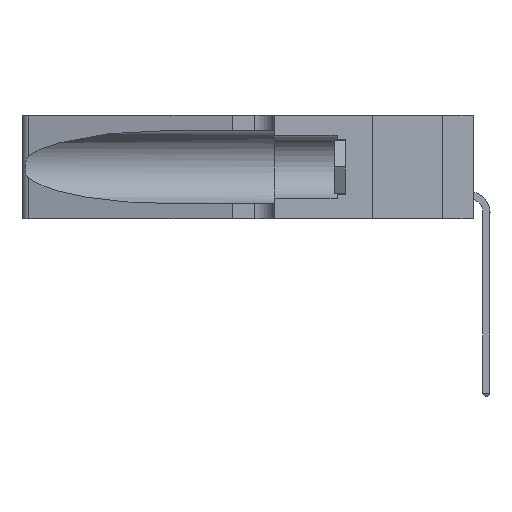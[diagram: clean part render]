
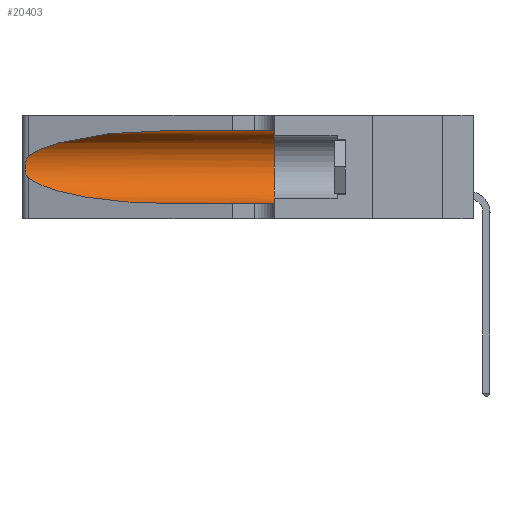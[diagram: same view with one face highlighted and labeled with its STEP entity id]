
A CAD part, left-side view. The second image highlights one B-rep face of the part: STEP entity #20403.
In plain terms, the highlighted cylindrical face has radius 3.308 mm (diameter 6.617 mm), a partial arc.
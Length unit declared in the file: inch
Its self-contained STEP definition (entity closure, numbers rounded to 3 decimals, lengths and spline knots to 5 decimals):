
#1357 = CARTESIAN_POINT ( 'NONE',  ( 0.1305, 1.61858, 0.31525 ) ) ;
#1443 =( BOUNDED_CURVE ( )  B_SPLINE_CURVE ( 3, ( #39841, #32537, #13638, #20014 ),
 .UNSPECIFIED., .F., .F. ) 
 B_SPLINE_CURVE_WITH_KNOTS ( ( 4, 4 ),
 ( 3.44316, 4.71239 ),
 .UNSPECIFIED. ) 
 CURVE ( )  GEOMETRIC_REPRESENTATION_ITEM ( )  RATIONAL_B_SPLINE_CURVE ( ( 1., 0.87, 0.87, 1. ) ) 
 REPRESENTATION_ITEM ( '' )  );
#2177 = DIRECTION ( 'NONE',  ( 0., -1., 0. ) ) ;
#2722 = CARTESIAN_POINT ( 'NONE',  ( 0.2373, 1.15595, 0.28018 ) ) ;
#2721 = CARTESIAN_POINT ( 'NONE',  ( 0.1305, 1.61858, 0.05475 ) ) ;
#4107 = EDGE_CURVE ( 'NONE', #25754, #6653, #5802, .T. ) ;
#4932 = VECTOR ( 'NONE', #26625, 39.37008 ) ;
#5802 =( BOUNDED_CURVE ( )  B_SPLINE_CURVE ( 3, ( #9171, #18716, #2722, #34427 ),
 .UNSPECIFIED., .F., .T. ) 
 B_SPLINE_CURVE_WITH_KNOTS ( ( 4, 4 ),
 ( 1.5708, 2.84003 ),
 .UNSPECIFIED. ) 
 CURVE ( )  GEOMETRIC_REPRESENTATION_ITEM ( )  RATIONAL_B_SPLINE_CURVE ( ( 1., 0.87, 0.87, 1. ) ) 
 REPRESENTATION_ITEM ( '' )  );
#6556 = CARTESIAN_POINT ( 'NONE',  ( 0.25639, 1.23186, 0.15144 ) ) ;
#6653 = VERTEX_POINT ( 'NONE', #25644 ) ;
#8670 = CARTESIAN_POINT ( 'NONE',  ( 0.26018, 1.23835, 0.19895 ) ) ;
#8811 = CARTESIAN_POINT ( 'NONE',  ( 0.26075, 1.23896, 0.178 ) ) ;
#8967 = AXIS2_PLACEMENT_3D ( 'NONE', #35806, #18061, #27048 ) ;
#9171 = CARTESIAN_POINT ( 'NONE',  ( 0.1305, 0.72297, 0.31525 ) ) ;
#10238 = CARTESIAN_POINT ( 'NONE',  ( 0.1305, 0.72297, 0.05475 ) ) ;
#13269 = LINE ( 'NONE', #1357, #4932 ) ;
#13638 = CARTESIAN_POINT ( 'NONE',  ( 0.18966, 0.96281, 0.05475 ) ) ;
#14385 = EDGE_CURVE ( 'NONE', #25754, #19859, #13269, .T. ) ;
#15028 = CARTESIAN_POINT ( 'NONE',  ( 0.25787, 1.23484, 0.2124 ) ) ;
#15361 = VERTEX_POINT ( 'NONE', #16841 ) ;
#16841 = CARTESIAN_POINT ( 'NONE',  ( 0.25487, 1.22718, 0.14631 ) ) ;
#18061 = DIRECTION ( 'NONE',  ( 0., 1., 0. ) ) ;
#18066 = CIRCLE ( 'NONE', #8967, 0.13025 ) ;
#18219 = CARTESIAN_POINT ( 'NONE',  ( 0.25854, 1.2359, 0.20912 ) ) ;
#18716 = CARTESIAN_POINT ( 'NONE',  ( 0.18966, 0.96281, 0.31525 ) ) ;
#19280 = CARTESIAN_POINT ( 'NONE',  ( 0.26017, 1.23833, 0.17102 ) ) ;
#19776 = LINE ( 'NONE', #2721, #21796 ) ;
#19859 = VERTEX_POINT ( 'NONE', #22447 ) ;
#20014 = CARTESIAN_POINT ( 'NONE',  ( 0.1305, 0.72297, 0.05475 ) ) ;
#20132 = EDGE_CURVE ( 'NONE', #30027, #28271, #19776, .T. ) ;
#20403 = ADVANCED_FACE ( 'NONE', ( #26137 ), #40463, .F. ) ;
#21622 = DIRECTION ( 'NONE',  ( 0., -1., 0. ) ) ;
#21796 = VECTOR ( 'NONE', #21622, 39.37008 ) ;
#22447 = CARTESIAN_POINT ( 'NONE',  ( 0.1305, 0.35, 0.31525 ) ) ;
#22456 = CARTESIAN_POINT ( 'NONE',  ( 0.25789, 1.23486, 0.15765 ) ) ;
#22770 = CARTESIAN_POINT ( 'NONE',  ( 0.1305, 0.35, 0.05475 ) ) ;
#23377 = ORIENTED_EDGE ( 'NONE', *, *, #30565, .T. ) ;
#24425 = CARTESIAN_POINT ( 'NONE',  ( 0.25639, 1.23184, 0.21858 ) ) ;
#24553 = CARTESIAN_POINT ( 'NONE',  ( 0.26075, 1.23896, 0.19203 ) ) ;
#25644 = CARTESIAN_POINT ( 'NONE',  ( 0.25487, 1.22718, 0.22369 ) ) ;
#25754 = VERTEX_POINT ( 'NONE', #32259 ) ;
#25926 = ORIENTED_EDGE ( 'NONE', *, *, #4107, .T. ) ;
#26137 = FACE_OUTER_BOUND ( 'NONE', #34894, .T. ) ;
#26625 = DIRECTION ( 'NONE',  ( 0., -1., 0. ) ) ;
#27048 = DIRECTION ( 'NONE',  ( 0., 0., 1. ) ) ;
#28271 = VERTEX_POINT ( 'NONE', #22770 ) ;
#28649 = CARTESIAN_POINT ( 'NONE',  ( 0.25487, 1.22718, 0.14631 ) ) ;
#28784 = CARTESIAN_POINT ( 'NONE',  ( 0.25555, 1.22993, 0.14849 ) ) ;
#30027 = VERTEX_POINT ( 'NONE', #10238 ) ;
#30565 = EDGE_CURVE ( 'NONE', #6653, #15361, #33834, .T. ) ;
#31299 = CARTESIAN_POINT ( 'NONE',  ( 0.25487, 1.22718, 0.22369 ) ) ;
#31335 = ORIENTED_EDGE ( 'NONE', *, *, #33545, .F. ) ;
#31791 = CARTESIAN_POINT ( 'NONE',  ( 0.25856, 1.23593, 0.16098 ) ) ;
#32259 = CARTESIAN_POINT ( 'NONE',  ( 0.1305, 0.72297, 0.31525 ) ) ;
#32537 = CARTESIAN_POINT ( 'NONE',  ( 0.2373, 1.15595, 0.08982 ) ) ;
#33545 = EDGE_CURVE ( 'NONE', #19859, #28271, #18066, .T. ) ;
#33834 = B_SPLINE_CURVE_WITH_KNOTS ( 'NONE', 3,
 ( #31299, #36942, #24425, #15028, #18219, #8670, #24553, #8811, #19280, #31791, #22456, #6556, #28784, #28649 ),
 .UNSPECIFIED., .F., .F.,
 ( 4, 2, 2, 2, 2, 2, 4 ),
 ( 0., 0.00027, 0.00053, 0.00107, 0.0016, 0.00187, 0.00214 ),
 .UNSPECIFIED. ) ;
#33987 = ORIENTED_EDGE ( 'NONE', *, *, #20132, .T. ) ;
#34271 = ORIENTED_EDGE ( 'NONE', *, *, #14385, .F. ) ;
#34427 = CARTESIAN_POINT ( 'NONE',  ( 0.25487, 1.22718, 0.22369 ) ) ;
#34894 = EDGE_LOOP ( 'NONE', ( #25926, #23377, #35706, #33987, #31335, #34271 ) ) ;
#35031 = AXIS2_PLACEMENT_3D ( 'NONE', #35933, #2177, #40213 ) ;
#35706 = ORIENTED_EDGE ( 'NONE', *, *, #37576, .T. ) ;
#35806 = CARTESIAN_POINT ( 'NONE',  ( 0.1305, 0.35, 0.185 ) ) ;
#35933 = CARTESIAN_POINT ( 'NONE',  ( 0.1305, 1.61858, 0.185 ) ) ;
#36942 = CARTESIAN_POINT ( 'NONE',  ( 0.25555, 1.22994, 0.2215 ) ) ;
#37576 = EDGE_CURVE ( 'NONE', #15361, #30027, #1443, .T. ) ;
#39841 = CARTESIAN_POINT ( 'NONE',  ( 0.25487, 1.22718, 0.14631 ) ) ;
#40213 = DIRECTION ( 'NONE',  ( 0., 0., -1. ) ) ;
#40463 = CYLINDRICAL_SURFACE ( 'NONE', #35031, 0.13025 ) ;
